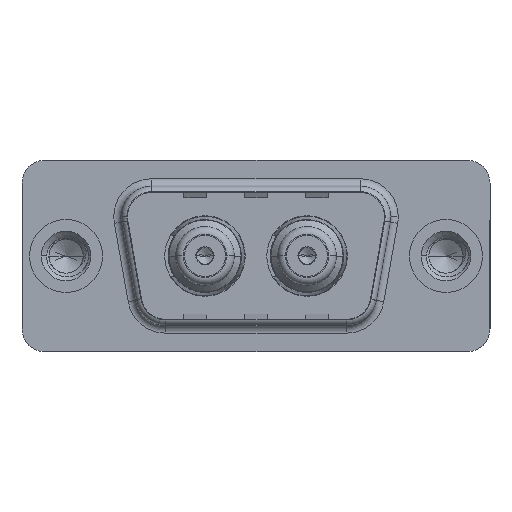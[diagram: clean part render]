
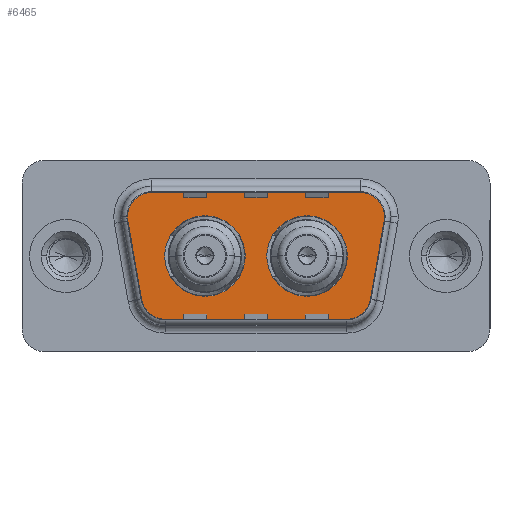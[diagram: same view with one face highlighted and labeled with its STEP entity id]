
A CAD part, top view. The second image highlights one B-rep face of the part: STEP entity #6465.
In plain terms, the highlighted planar face has unit normal (0, 0, 1).
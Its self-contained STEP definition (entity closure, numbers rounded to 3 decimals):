
#23 = VERTEX_POINT ( 'NONE', #5565 ) ;
#42 = CARTESIAN_POINT ( 'NONE',  ( 9.14, 0., 0. ) ) ;
#160 = CIRCLE ( 'NONE', #673, 2.65 ) ;
#163 = AXIS2_PLACEMENT_3D ( 'NONE', #4685, #12640, #5869 ) ;
#314 = AXIS2_PLACEMENT_3D ( 'NONE', #3747, #11679, #10702 ) ;
#434 = CARTESIAN_POINT ( 'NONE',  ( 19.564, 4.9, 0. ) ) ;
#673 = AXIS2_PLACEMENT_3D ( 'NONE', #42, #8361, #1278 ) ;
#801 = VERTEX_POINT ( 'NONE', #12097 ) ;
#865 = VECTOR ( 'NONE', #9593, 1000. ) ;
#896 = EDGE_LOOP ( 'NONE', ( #6339, #2099, #5491, #6542, #11003, #9430, #5863, #2503, #6744 ) ) ;
#1077 = VERTEX_POINT ( 'NONE', #5302 ) ;
#1080 = EDGE_CURVE ( 'NONE', #23, #11179, #13532, .T. ) ;
#1278 = DIRECTION ( 'NONE',  ( 1., 0., 0. ) ) ;
#1288 = VERTEX_POINT ( 'NONE', #2689 ) ;
#1360 = DIRECTION ( 'NONE',  ( 0., 0., 1. ) ) ;
#1609 = VERTEX_POINT ( 'NONE', #13266 ) ;
#1795 = VERTEX_POINT ( 'NONE', #7887 ) ;
#2002 = DIRECTION ( 'NONE',  ( 0.174, -0.985, 0. ) ) ;
#2004 = DIRECTION ( 'NONE',  ( 1., 0., 0. ) ) ;
#2099 = ORIENTED_EDGE ( 'NONE', *, *, #13803, .T. ) ;
#2154 = EDGE_CURVE ( 'NONE', #8584, #4113, #14216, .T. ) ;
#2416 = CARTESIAN_POINT ( 'NONE',  ( 21.534, 2.553, 0. ) ) ;
#2490 = FACE_OUTER_BOUND ( 'NONE', #896, .T. ) ;
#2503 = ORIENTED_EDGE ( 'NONE', *, *, #5606, .T. ) ;
#2541 = DIRECTION ( 'NONE',  ( 0., 0., 1. ) ) ;
#2627 = VERTEX_POINT ( 'NONE', #9213 ) ;
#2689 = CARTESIAN_POINT ( 'NONE',  ( 6.49, 0., 0. ) ) ;
#2726 = CARTESIAN_POINT ( 'NONE',  ( 3.466, 2.553, 0. ) ) ;
#2873 = CIRCLE ( 'NONE', #314, 2. ) ;
#3009 = ORIENTED_EDGE ( 'NONE', *, *, #3039, .F. ) ;
#3039 = EDGE_CURVE ( 'NONE', #801, #1288, #7557, .T. ) ;
#3080 = CIRCLE ( 'NONE', #13347, 2. ) ;
#3397 = CIRCLE ( 'NONE', #13563, 2.65 ) ;
#3399 = CARTESIAN_POINT ( 'NONE',  ( 6.459, -4.9, 0. ) ) ;
#3449 = AXIS2_PLACEMENT_3D ( 'NONE', #8062, #4665, #2004 ) ;
#3585 = CARTESIAN_POINT ( 'NONE',  ( 21.534, 2.553, 0. ) ) ;
#3747 = CARTESIAN_POINT ( 'NONE',  ( 5.436, 2.9, 0. ) ) ;
#4021 = DIRECTION ( 'NONE',  ( 1., 0., 0. ) ) ;
#4113 = VERTEX_POINT ( 'NONE', #8798 ) ;
#4447 = VERTEX_POINT ( 'NONE', #2726 ) ;
#4665 = DIRECTION ( 'NONE',  ( 0., 0., 1. ) ) ;
#4685 = CARTESIAN_POINT ( 'NONE',  ( 18.541, -2.9, 0. ) ) ;
#4781 = CIRCLE ( 'NONE', #6250, 2.65 ) ;
#5275 = ORIENTED_EDGE ( 'NONE', *, *, #7975, .F. ) ;
#5302 = CARTESIAN_POINT ( 'NONE',  ( 18.51, 0., 0. ) ) ;
#5441 = VECTOR ( 'NONE', #2002, 1000. ) ;
#5491 = ORIENTED_EDGE ( 'NONE', *, *, #2154, .T. ) ;
#5526 = AXIS2_PLACEMENT_3D ( 'NONE', #7499, #10320, #14309 ) ;
#5565 = CARTESIAN_POINT ( 'NONE',  ( 6.459, -4.9, 0. ) ) ;
#5572 = CARTESIAN_POINT ( 'NONE',  ( 3.466, 2.553, 0. ) ) ;
#5606 = EDGE_CURVE ( 'NONE', #1795, #23, #3080, .T. ) ;
#5688 = DIRECTION ( 'NONE',  ( -1., 0., 0. ) ) ;
#5763 = EDGE_CURVE ( 'NONE', #1077, #2627, #4781, .T. ) ;
#5863 = ORIENTED_EDGE ( 'NONE', *, *, #9877, .T. ) ;
#5869 = DIRECTION ( 'NONE',  ( 1., 0., 0. ) ) ;
#5939 = EDGE_CURVE ( 'NONE', #1609, #4447, #2873, .T. ) ;
#5973 = ORIENTED_EDGE ( 'NONE', *, *, #5763, .F. ) ;
#6165 = DIRECTION ( 'NONE',  ( 0., 0., 1. ) ) ;
#6250 = AXIS2_PLACEMENT_3D ( 'NONE', #11321, #11197, #7903 ) ;
#6339 = ORIENTED_EDGE ( 'NONE', *, *, #13689, .T. ) ;
#6367 = AXIS2_PLACEMENT_3D ( 'NONE', #12945, #6165, #14068 ) ;
#6465 = ADVANCED_FACE ( 'NONE', ( #14743, #11360, #2490 ), #14755, .T. ) ;
#6481 = LINE ( 'NONE', #2416, #14478 ) ;
#6542 = ORIENTED_EDGE ( 'NONE', *, *, #10870, .T. ) ;
#6744 = ORIENTED_EDGE ( 'NONE', *, *, #1080, .T. ) ;
#6827 = CARTESIAN_POINT ( 'NONE',  ( 20.511, -3.247, 0. ) ) ;
#6938 = AXIS2_PLACEMENT_3D ( 'NONE', #10307, #10901, #4021 ) ;
#7192 = CARTESIAN_POINT ( 'NONE',  ( 5.436, 4.9, 0. ) ) ;
#7499 = CARTESIAN_POINT ( 'NONE',  ( 19.564, 2.9, 0. ) ) ;
#7557 = CIRCLE ( 'NONE', #3449, 2.65 ) ;
#7887 = CARTESIAN_POINT ( 'NONE',  ( 4.489, -3.247, 0. ) ) ;
#7903 = DIRECTION ( 'NONE',  ( 1., 0., 0. ) ) ;
#7949 = VECTOR ( 'NONE', #8308, 1000. ) ;
#7975 = EDGE_CURVE ( 'NONE', #1288, #801, #160, .T. ) ;
#8062 = CARTESIAN_POINT ( 'NONE',  ( 9.14, 0., 0. ) ) ;
#8308 = DIRECTION ( 'NONE',  ( -1., 0., 0. ) ) ;
#8361 = DIRECTION ( 'NONE',  ( 0., 0., 1. ) ) ;
#8457 = VERTEX_POINT ( 'NONE', #6827 ) ;
#8584 = VERTEX_POINT ( 'NONE', #3585 ) ;
#8643 = EDGE_CURVE ( 'NONE', #2627, #1077, #3397, .T. ) ;
#8798 = CARTESIAN_POINT ( 'NONE',  ( 21.564, 2.9, 0. ) ) ;
#9213 = CARTESIAN_POINT ( 'NONE',  ( 13.21, 0., 0. ) ) ;
#9430 = ORIENTED_EDGE ( 'NONE', *, *, #5939, .T. ) ;
#9520 = CARTESIAN_POINT ( 'NONE',  ( 15.86, 0., 0. ) ) ;
#9593 = DIRECTION ( 'NONE',  ( 1., 0., 0. ) ) ;
#9733 = VERTEX_POINT ( 'NONE', #434 ) ;
#9877 = EDGE_CURVE ( 'NONE', #4447, #1795, #11466, .T. ) ;
#10134 = EDGE_CURVE ( 'NONE', #9733, #1609, #11295, .T. ) ;
#10235 = CARTESIAN_POINT ( 'NONE',  ( 18.541, -4.9, 0. ) ) ;
#10307 = CARTESIAN_POINT ( 'NONE',  ( 18.541, -2.9, 0. ) ) ;
#10320 = DIRECTION ( 'NONE',  ( 0., 0., 1. ) ) ;
#10627 = DIRECTION ( 'NONE',  ( 1., 0., 0. ) ) ;
#10702 = DIRECTION ( 'NONE',  ( 1., 0., 0. ) ) ;
#10870 = EDGE_CURVE ( 'NONE', #4113, #9733, #11190, .T. ) ;
#10901 = DIRECTION ( 'NONE',  ( 0., 0., 1. ) ) ;
#11003 = ORIENTED_EDGE ( 'NONE', *, *, #10134, .T. ) ;
#11179 = VERTEX_POINT ( 'NONE', #10235 ) ;
#11190 = CIRCLE ( 'NONE', #6367, 2. ) ;
#11197 = DIRECTION ( 'NONE',  ( 0., 0., 1. ) ) ;
#11295 = LINE ( 'NONE', #7192, #7949 ) ;
#11321 = CARTESIAN_POINT ( 'NONE',  ( 15.86, 0., 0. ) ) ;
#11360 = FACE_BOUND ( 'NONE', #14000, .T. ) ;
#11466 = LINE ( 'NONE', #5572, #5441 ) ;
#11474 = EDGE_LOOP ( 'NONE', ( #5973, #13408 ) ) ;
#11679 = DIRECTION ( 'NONE',  ( 0., 0., 1. ) ) ;
#12097 = CARTESIAN_POINT ( 'NONE',  ( 11.79, 0., 0. ) ) ;
#12521 = CIRCLE ( 'NONE', #163, 2. ) ;
#12640 = DIRECTION ( 'NONE',  ( 0., 0., 1. ) ) ;
#12945 = CARTESIAN_POINT ( 'NONE',  ( 19.564, 2.9, 0. ) ) ;
#13266 = CARTESIAN_POINT ( 'NONE',  ( 5.436, 4.9, 0. ) ) ;
#13347 = AXIS2_PLACEMENT_3D ( 'NONE', #13901, #1360, #5688 ) ;
#13408 = ORIENTED_EDGE ( 'NONE', *, *, #8643, .F. ) ;
#13532 = LINE ( 'NONE', #3399, #865 ) ;
#13563 = AXIS2_PLACEMENT_3D ( 'NONE', #9520, #2541, #10627 ) ;
#13689 = EDGE_CURVE ( 'NONE', #11179, #8457, #12521, .T. ) ;
#13803 = EDGE_CURVE ( 'NONE', #8457, #8584, #6481, .T. ) ;
#13901 = CARTESIAN_POINT ( 'NONE',  ( 6.459, -2.9, 0. ) ) ;
#14000 = EDGE_LOOP ( 'NONE', ( #3009, #5275 ) ) ;
#14068 = DIRECTION ( 'NONE',  ( -1., 0., 0. ) ) ;
#14216 = CIRCLE ( 'NONE', #5526, 2. ) ;
#14309 = DIRECTION ( 'NONE',  ( -1., 0., 0. ) ) ;
#14478 = VECTOR ( 'NONE', #15056, 1000. ) ;
#14743 = FACE_BOUND ( 'NONE', #11474, .T. ) ;
#14755 = PLANE ( 'NONE',  #6938 ) ;
#15056 = DIRECTION ( 'NONE',  ( 0.174, 0.985, 0. ) ) ;
